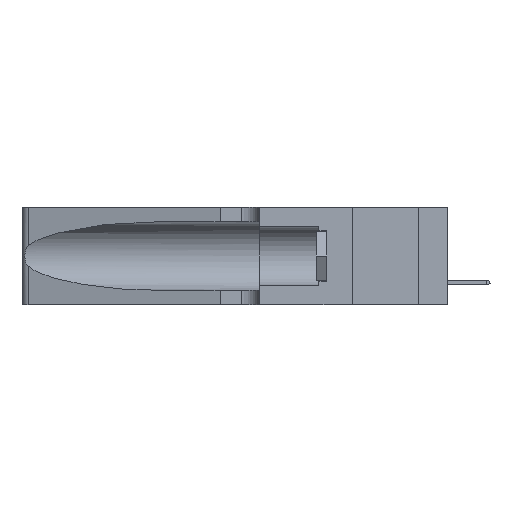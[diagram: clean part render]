
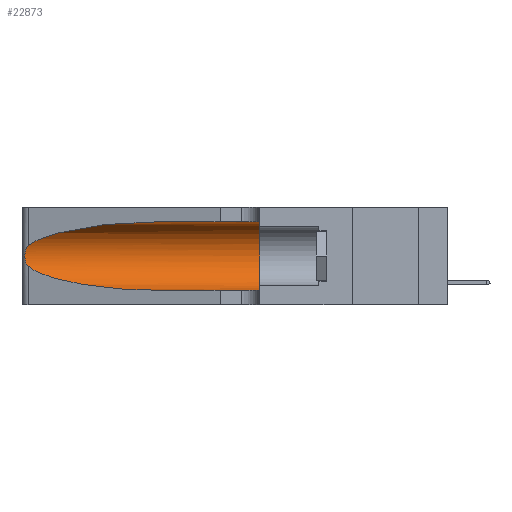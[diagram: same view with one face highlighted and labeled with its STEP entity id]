
A CAD part, left-side view. The second image highlights one B-rep face of the part: STEP entity #22873.
In plain terms, the highlighted cylindrical face has radius 3.308 mm (diameter 6.617 mm), a partial arc.
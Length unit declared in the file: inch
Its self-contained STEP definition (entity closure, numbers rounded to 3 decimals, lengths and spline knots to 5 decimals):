
#133 = EDGE_LOOP ( 'NONE', ( #16374, #20851, #18609, #24599, #2178, #33786 ) ) ;
#385 = CARTESIAN_POINT ( 'NONE',  ( 0.18966, 0.96281, 0.05475 ) ) ;
#1509 = CARTESIAN_POINT ( 'NONE',  ( 0.1305, 1.61858, 0.31525 ) ) ;
#1811 = CARTESIAN_POINT ( 'NONE',  ( 0.26075, 1.23896, 0.19203 ) ) ;
#1934 = CARTESIAN_POINT ( 'NONE',  ( 0.25856, 1.23593, 0.16098 ) ) ;
#2178 = ORIENTED_EDGE ( 'NONE', *, *, #35575, .F. ) ;
#2832 = CARTESIAN_POINT ( 'NONE',  ( 0.2373, 1.15595, 0.28018 ) ) ;
#3046 = CARTESIAN_POINT ( 'NONE',  ( 0.1305, 0.72297, 0.05475 ) ) ;
#4007 =( BOUNDED_CURVE ( )  B_SPLINE_CURVE ( 3, ( #25411, #5944, #385, #3046 ),
 .UNSPECIFIED., .F., .T. ) 
 B_SPLINE_CURVE_WITH_KNOTS ( ( 4, 4 ),
 ( 3.44316, 4.71239 ),
 .UNSPECIFIED. ) 
 CURVE ( )  GEOMETRIC_REPRESENTATION_ITEM ( )  RATIONAL_B_SPLINE_CURVE ( ( 1., 0.87, 0.87, 1. ) ) 
 REPRESENTATION_ITEM ( '' )  );
#4858 = CARTESIAN_POINT ( 'NONE',  ( 0.26018, 1.23835, 0.19895 ) ) ;
#5944 = CARTESIAN_POINT ( 'NONE',  ( 0.2373, 1.15595, 0.08982 ) ) ;
#6064 = DIRECTION ( 'NONE',  ( 0., 0., 1. ) ) ;
#6528 = CARTESIAN_POINT ( 'NONE',  ( 0.25639, 1.23184, 0.21858 ) ) ;
#7067 = DIRECTION ( 'NONE',  ( 0., -1., 0. ) ) ;
#7259 = EDGE_CURVE ( 'NONE', #20656, #35681, #4007, .T. ) ;
#7671 = CARTESIAN_POINT ( 'NONE',  ( 0.25789, 1.23486, 0.15765 ) ) ;
#7972 = CARTESIAN_POINT ( 'NONE',  ( 0.25487, 1.22718, 0.22369 ) ) ;
#9571 = CARTESIAN_POINT ( 'NONE',  ( 0.25555, 1.22994, 0.2215 ) ) ;
#9588 = LINE ( 'NONE', #1509, #35551 ) ;
#9814 = VERTEX_POINT ( 'NONE', #7972 ) ;
#9977 = EDGE_CURVE ( 'NONE', #14075, #9814, #20672, .T. ) ;
#10646 = CARTESIAN_POINT ( 'NONE',  ( 0.25487, 1.22718, 0.14631 ) ) ;
#11079 = CARTESIAN_POINT ( 'NONE',  ( 0.1305, 0.72297, 0.31525 ) ) ;
#13218 = VERTEX_POINT ( 'NONE', #29887 ) ;
#13385 = DIRECTION ( 'NONE',  ( 0., -1., 0. ) ) ;
#13454 = CARTESIAN_POINT ( 'NONE',  ( 0.25487, 1.22718, 0.14631 ) ) ;
#13568 = CARTESIAN_POINT ( 'NONE',  ( 0.25555, 1.22993, 0.14849 ) ) ;
#13639 = CARTESIAN_POINT ( 'NONE',  ( 0.18966, 0.96281, 0.31525 ) ) ;
#14075 = VERTEX_POINT ( 'NONE', #31747 ) ;
#15402 = CARTESIAN_POINT ( 'NONE',  ( 0.25787, 1.23484, 0.2124 ) ) ;
#15541 = CARTESIAN_POINT ( 'NONE',  ( 0.26017, 1.23833, 0.17102 ) ) ;
#15774 = CARTESIAN_POINT ( 'NONE',  ( 0.26075, 1.23896, 0.178 ) ) ;
#16374 = ORIENTED_EDGE ( 'NONE', *, *, #9977, .T. ) ;
#16672 = DIRECTION ( 'NONE',  ( 0., -1., 0. ) ) ;
#18060 = EDGE_CURVE ( 'NONE', #14075, #28618, #9588, .T. ) ;
#18103 = EDGE_CURVE ( 'NONE', #9814, #20656, #20213, .T. ) ;
#18456 = CIRCLE ( 'NONE', #31255, 0.13025 ) ;
#18609 = ORIENTED_EDGE ( 'NONE', *, *, #7259, .T. ) ;
#19669 = CARTESIAN_POINT ( 'NONE',  ( 0.1305, 1.61858, 0.05475 ) ) ;
#20213 = B_SPLINE_CURVE_WITH_KNOTS ( 'NONE', 3,
 ( #26118, #9571, #6528, #15402, #25876, #4858, #1811, #15774, #15541, #1934, #7671, #26608, #13568, #13454 ),
 .UNSPECIFIED., .F., .F.,
 ( 4, 2, 2, 2, 2, 2, 4 ),
 ( 0., 0.00027, 0.00053, 0.00107, 0.0016, 0.00187, 0.00214 ),
 .UNSPECIFIED. ) ;
#20656 = VERTEX_POINT ( 'NONE', #10646 ) ;
#20672 =( BOUNDED_CURVE ( )  B_SPLINE_CURVE ( 3, ( #11079, #13639, #2832, #32964 ),
 .UNSPECIFIED., .F., .T. ) 
 B_SPLINE_CURVE_WITH_KNOTS ( ( 4, 4 ),
 ( 1.5708, 2.84003 ),
 .UNSPECIFIED. ) 
 CURVE ( )  GEOMETRIC_REPRESENTATION_ITEM ( )  RATIONAL_B_SPLINE_CURVE ( ( 1., 0.87, 0.87, 1. ) ) 
 REPRESENTATION_ITEM ( '' )  );
#20851 = ORIENTED_EDGE ( 'NONE', *, *, #18103, .T. ) ;
#21740 = DIRECTION ( 'NONE',  ( 0., 0., -1. ) ) ;
#21961 = FACE_OUTER_BOUND ( 'NONE', #133, .T. ) ;
#22873 = ADVANCED_FACE ( 'NONE', ( #21961 ), #23674, .F. ) ;
#22905 = CARTESIAN_POINT ( 'NONE',  ( 0.1305, 0.72297, 0.05475 ) ) ;
#23674 = CYLINDRICAL_SURFACE ( 'NONE', #30785, 0.13025 ) ;
#24599 = ORIENTED_EDGE ( 'NONE', *, *, #34624, .T. ) ;
#24753 = CARTESIAN_POINT ( 'NONE',  ( 0.1305, 1.61858, 0.185 ) ) ;
#25411 = CARTESIAN_POINT ( 'NONE',  ( 0.25487, 1.22718, 0.14631 ) ) ;
#25422 = DIRECTION ( 'NONE',  ( 0., 1., 0. ) ) ;
#25876 = CARTESIAN_POINT ( 'NONE',  ( 0.25854, 1.2359, 0.20912 ) ) ;
#26118 = CARTESIAN_POINT ( 'NONE',  ( 0.25487, 1.22718, 0.22369 ) ) ;
#26608 = CARTESIAN_POINT ( 'NONE',  ( 0.25639, 1.23186, 0.15144 ) ) ;
#28425 = LINE ( 'NONE', #19669, #28833 ) ;
#28618 = VERTEX_POINT ( 'NONE', #28636 ) ;
#28636 = CARTESIAN_POINT ( 'NONE',  ( 0.1305, 0.35, 0.31525 ) ) ;
#28833 = VECTOR ( 'NONE', #16672, 39.37008 ) ;
#29887 = CARTESIAN_POINT ( 'NONE',  ( 0.1305, 0.35, 0.05475 ) ) ;
#30785 = AXIS2_PLACEMENT_3D ( 'NONE', #24753, #13385, #21740 ) ;
#31255 = AXIS2_PLACEMENT_3D ( 'NONE', #31345, #25422, #6064 ) ;
#31345 = CARTESIAN_POINT ( 'NONE',  ( 0.1305, 0.35, 0.185 ) ) ;
#31747 = CARTESIAN_POINT ( 'NONE',  ( 0.1305, 0.72297, 0.31525 ) ) ;
#32964 = CARTESIAN_POINT ( 'NONE',  ( 0.25487, 1.22718, 0.22369 ) ) ;
#33786 = ORIENTED_EDGE ( 'NONE', *, *, #18060, .F. ) ;
#34624 = EDGE_CURVE ( 'NONE', #35681, #13218, #28425, .T. ) ;
#35551 = VECTOR ( 'NONE', #7067, 39.37008 ) ;
#35575 = EDGE_CURVE ( 'NONE', #28618, #13218, #18456, .T. ) ;
#35681 = VERTEX_POINT ( 'NONE', #22905 ) ;
